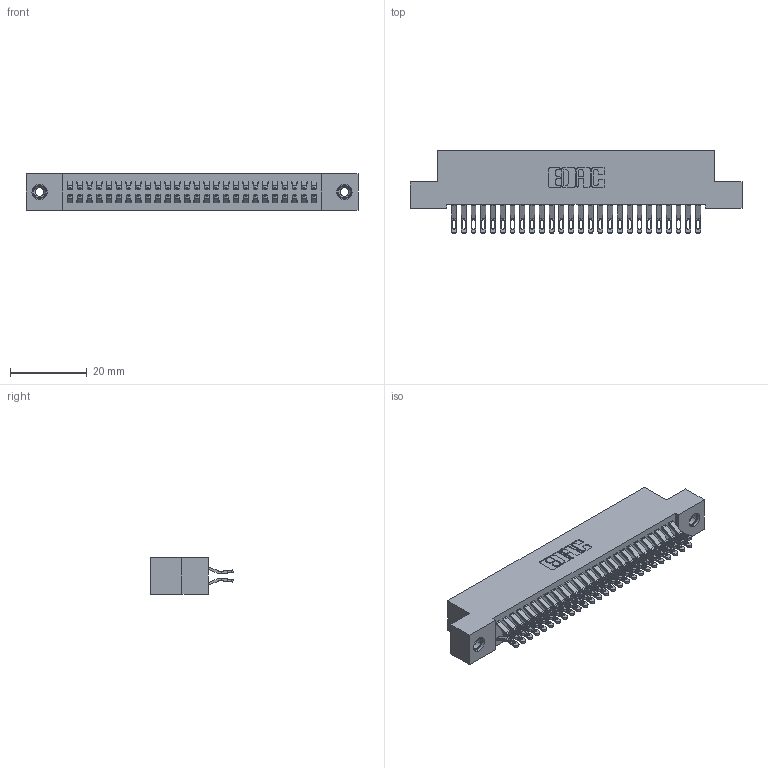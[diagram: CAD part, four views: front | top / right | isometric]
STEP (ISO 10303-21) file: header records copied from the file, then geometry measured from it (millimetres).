
FILE_DESCRIPTION (( 'STEP AP203' ), '1' );
FILE_NAME ('392-052-555-208.STEP', '2019-10-08T12:46:58', ( '' ), ( '' ), 'SwSTEP 2.0', 'SolidWorks 2016', '' );
FILE_SCHEMA (( 'CONFIG_CONTROL_DESIGN' ));
Length unit declared in the file: inch
Products named in the file (4): 342 Part_TI; 345-292-001_555 Tail; 345-250-001_345-250-003-102; 392-052-555-208
Assembly tree (55 placements, depth 2):
  392-052-555-208
    342 Part_TI
    345-292-001_555 Tail  x52
    345-250-001_345-250-003-102  x2
Bounding box: 86.36 x 21.47 x 9.4 mm (x, y, z)
Volume: 7822.5 mm3; surface area: 12852.3 mm2
Topology: 55 solids, 55 shells, 3186 faces, 9951 edges, 6626 vertices
Faces by surface type: plane 1866, cylinder 1304, cone 12, torus 4
Entity records: 20176 total; most frequent: CARTESIAN_POINT 3379, ORIENTED_EDGE 3278, DIRECTION 2917, EDGE_CURVE 1639, LINE 1471, VECTOR 1471, VERTEX_POINT 1088, AXIS2_PLACEMENT_3D 723
